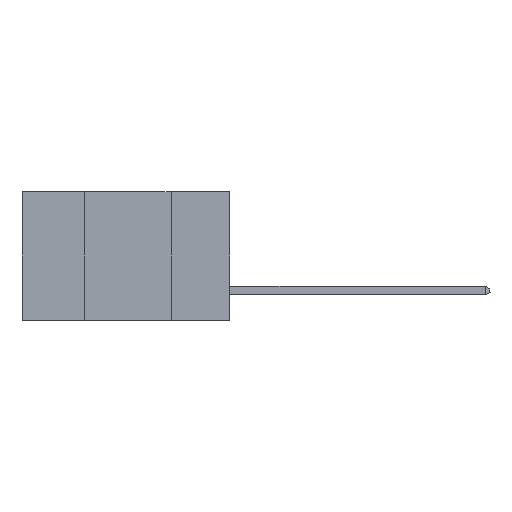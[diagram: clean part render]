
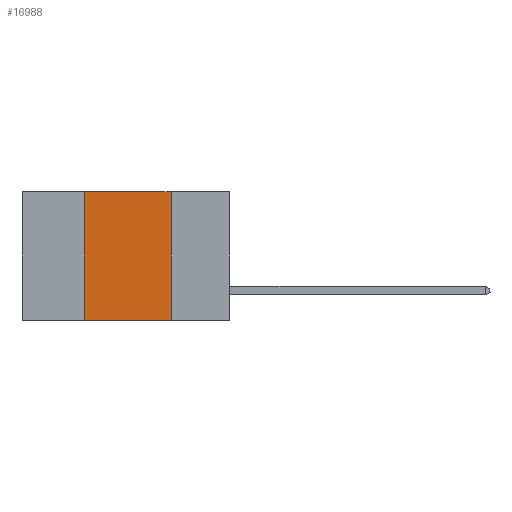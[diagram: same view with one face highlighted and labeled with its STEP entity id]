
A CAD part, left-side view. The second image highlights one B-rep face of the part: STEP entity #16988.
In plain terms, the highlighted planar face has unit normal (-1, 0, 0).
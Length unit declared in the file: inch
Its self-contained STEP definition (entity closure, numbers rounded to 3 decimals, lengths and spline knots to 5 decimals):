
#2724 = VERTEX_POINT ( 'NONE', #6472 ) ;
#2757 = EDGE_CURVE ( 'NONE', #15177, #2724, #3831, .T. ) ;
#3339 = CARTESIAN_POINT ( 'NONE',  ( 0., 0.42, 0. ) ) ;
#3750 = VECTOR ( 'NONE', #19785, 39.37008 ) ;
#3831 = LINE ( 'NONE', #13966, #15347 ) ;
#4485 = CARTESIAN_POINT ( 'NONE',  ( 0., 0.42, 0. ) ) ;
#5068 = DIRECTION ( 'NONE',  ( 1., 0., 0. ) ) ;
#6393 = CARTESIAN_POINT ( 'NONE',  ( 0., 0.17, 0. ) ) ;
#6472 = CARTESIAN_POINT ( 'NONE',  ( 0., 0.17, -0.37 ) ) ;
#6895 = DIRECTION ( 'NONE',  ( 0., 0., -1. ) ) ;
#7391 = CARTESIAN_POINT ( 'NONE',  ( 0., 0.17, 0. ) ) ;
#7550 = DIRECTION ( 'NONE',  ( 0., 0., -1. ) ) ;
#7659 = LINE ( 'NONE', #22819, #14598 ) ;
#7685 = FACE_OUTER_BOUND ( 'NONE', #9301, .T. ) ;
#7844 = LINE ( 'NONE', #7391, #22156 ) ;
#9301 = EDGE_LOOP ( 'NONE', ( #21591, #21858, #21341, #22396 ) ) ;
#9893 = DIRECTION ( 'NONE',  ( 0., -1., 0. ) ) ;
#13966 = CARTESIAN_POINT ( 'NONE',  ( 0., 0.6, -0.37 ) ) ;
#14105 = LINE ( 'NONE', #3339, #3750 ) ;
#14247 = EDGE_CURVE ( 'NONE', #21189, #2724, #7844, .T. ) ;
#14598 = VECTOR ( 'NONE', #22659, 39.37008 ) ;
#15177 = VERTEX_POINT ( 'NONE', #21013 ) ;
#15347 = VECTOR ( 'NONE', #9893, 39.37008 ) ;
#15615 = EDGE_CURVE ( 'NONE', #15177, #18751, #14105, .T. ) ;
#16068 = PLANE ( 'NONE',  #17823 ) ;
#16988 = ADVANCED_FACE ( 'NONE', ( #7685 ), #16068, .F. ) ;
#17316 = EDGE_CURVE ( 'NONE', #18751, #21189, #7659, .T. ) ;
#17823 = AXIS2_PLACEMENT_3D ( 'NONE', #18080, #5068, #6895 ) ;
#18080 = CARTESIAN_POINT ( 'NONE',  ( 0., 0.6, 0. ) ) ;
#18751 = VERTEX_POINT ( 'NONE', #4485 ) ;
#19785 = DIRECTION ( 'NONE',  ( 0., 0., 1. ) ) ;
#21013 = CARTESIAN_POINT ( 'NONE',  ( 0., 0.42, -0.37 ) ) ;
#21189 = VERTEX_POINT ( 'NONE', #6393 ) ;
#21341 = ORIENTED_EDGE ( 'NONE', *, *, #15615, .F. ) ;
#21591 = ORIENTED_EDGE ( 'NONE', *, *, #14247, .F. ) ;
#21858 = ORIENTED_EDGE ( 'NONE', *, *, #17316, .F. ) ;
#22156 = VECTOR ( 'NONE', #7550, 39.37008 ) ;
#22396 = ORIENTED_EDGE ( 'NONE', *, *, #2757, .T. ) ;
#22659 = DIRECTION ( 'NONE',  ( 0., -1., 0. ) ) ;
#22819 = CARTESIAN_POINT ( 'NONE',  ( 0., 0.6, 0. ) ) ;
